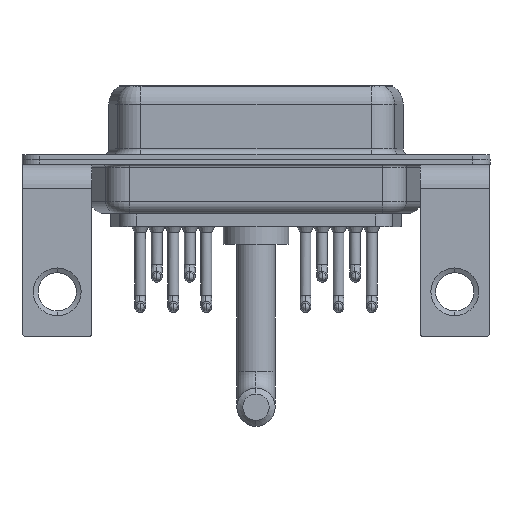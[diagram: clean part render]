
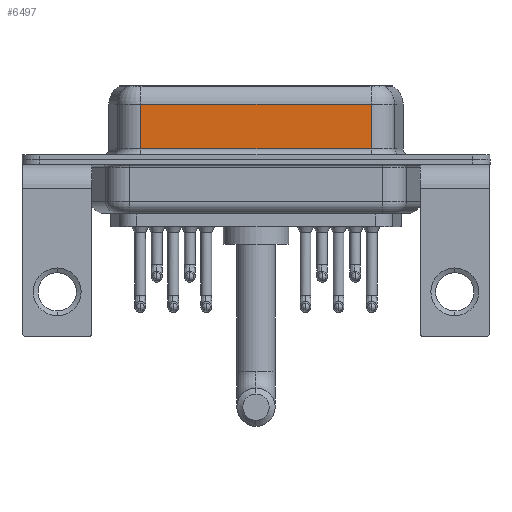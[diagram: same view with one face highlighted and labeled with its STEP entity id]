
A CAD part, front view. The second image highlights one B-rep face of the part: STEP entity #6497.
In plain terms, the highlighted planar face has unit normal (0, -1, 0).
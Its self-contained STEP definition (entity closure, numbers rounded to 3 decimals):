
#600 = VECTOR ( 'NONE', #10416, 1000. ) ;
#660 = DIRECTION ( 'NONE',  ( 0., 0., -1. ) ) ;
#784 = LINE ( 'NONE', #5305, #15584 ) ;
#2462 = EDGE_CURVE ( 'NONE', #8523, #3947, #12468, .T. ) ;
#3267 = CARTESIAN_POINT ( 'NONE',  ( 26.287, -3.95, 0.9 ) ) ;
#3947 = VERTEX_POINT ( 'NONE', #13933 ) ;
#4214 = ORIENTED_EDGE ( 'NONE', *, *, #15061, .F. ) ;
#4411 = LINE ( 'NONE', #6284, #600 ) ;
#4890 = CARTESIAN_POINT ( 'NONE',  ( 7.013, -3.95, 4.65 ) ) ;
#5173 = CARTESIAN_POINT ( 'NONE',  ( 7.013, -3.95, 6.4 ) ) ;
#5270 = VECTOR ( 'NONE', #660, 1000. ) ;
#5305 = CARTESIAN_POINT ( 'NONE',  ( 26.287, -3.95, 6.4 ) ) ;
#5725 = VERTEX_POINT ( 'NONE', #14974 ) ;
#6200 = EDGE_LOOP ( 'NONE', ( #4214, #13465, #14878, #12022 ) ) ;
#6283 = EDGE_CURVE ( 'NONE', #5725, #8523, #7568, .T. ) ;
#6284 = CARTESIAN_POINT ( 'NONE',  ( 26.287, -3.95, 0.9 ) ) ;
#6497 = ADVANCED_FACE ( 'NONE', ( #7076 ), #11313, .F. ) ;
#7076 = FACE_OUTER_BOUND ( 'NONE', #6200, .T. ) ;
#7447 = VECTOR ( 'NONE', #11693, 1000. ) ;
#7568 = LINE ( 'NONE', #13563, #7447 ) ;
#7896 = AXIS2_PLACEMENT_3D ( 'NONE', #11508, #12988, #13079 ) ;
#8523 = VERTEX_POINT ( 'NONE', #4890 ) ;
#10416 = DIRECTION ( 'NONE',  ( 1., 0., 0. ) ) ;
#11313 = PLANE ( 'NONE',  #7896 ) ;
#11508 = CARTESIAN_POINT ( 'NONE',  ( 26.287, -3.95, 6.4 ) ) ;
#11693 = DIRECTION ( 'NONE',  ( -1., 0., 0. ) ) ;
#12022 = ORIENTED_EDGE ( 'NONE', *, *, #17215, .T. ) ;
#12468 = LINE ( 'NONE', #5173, #5270 ) ;
#12988 = DIRECTION ( 'NONE',  ( 0., 1., 0. ) ) ;
#13079 = DIRECTION ( 'NONE',  ( 0., 0., 1. ) ) ;
#13465 = ORIENTED_EDGE ( 'NONE', *, *, #6283, .T. ) ;
#13563 = CARTESIAN_POINT ( 'NONE',  ( 26.287, -3.95, 4.65 ) ) ;
#13933 = CARTESIAN_POINT ( 'NONE',  ( 7.013, -3.95, 0.9 ) ) ;
#14878 = ORIENTED_EDGE ( 'NONE', *, *, #2462, .T. ) ;
#14974 = CARTESIAN_POINT ( 'NONE',  ( 26.287, -3.95, 4.65 ) ) ;
#15061 = EDGE_CURVE ( 'NONE', #5725, #15145, #784, .T. ) ;
#15145 = VERTEX_POINT ( 'NONE', #3267 ) ;
#15584 = VECTOR ( 'NONE', #18685, 1000. ) ;
#17215 = EDGE_CURVE ( 'NONE', #3947, #15145, #4411, .T. ) ;
#18685 = DIRECTION ( 'NONE',  ( 0., 0., -1. ) ) ;
